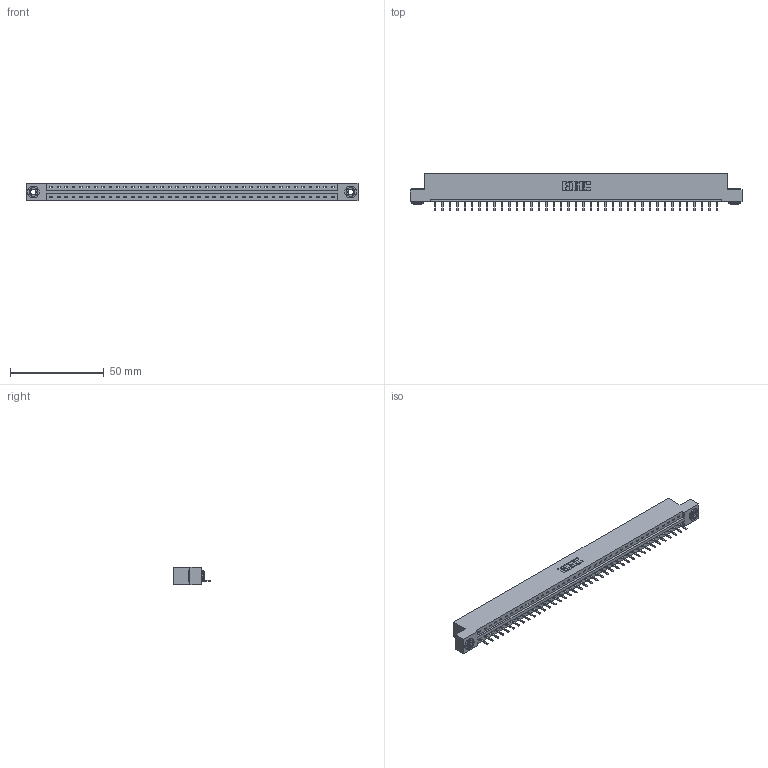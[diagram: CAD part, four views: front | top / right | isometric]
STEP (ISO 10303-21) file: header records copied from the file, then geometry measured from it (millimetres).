
FILE_DESCRIPTION (( 'STEP AP203' ), '1' );
FILE_NAME ('337-039-520-103.STEP', '2019-10-01T18:00:44', ( '' ), ( '' ), 'SwSTEP 2.0', 'SolidWorks 2016', '' );
FILE_SCHEMA (( 'CONFIG_CONTROL_DESIGN' ));
Length unit declared in the file: inch
Products named in the file (4): 345-292-001_345-293-120; 345-250-002_345-250-002-102; 337-039-520-103; 337 Part_Flush Mounting Lugs - 0.156 Dia-TH
Assembly tree (42 placements, depth 2):
  337-039-520-103
    337 Part_Flush Mounting Lugs - 0.156 Dia-TH
    345-292-001_345-293-120  x39
    345-250-002_345-250-002-102  x2
Bounding box: 177.55 x 20.02 x 9.4 mm (x, y, z)
Volume: 18322.6 mm3; surface area: 18745.9 mm2
Topology: 42 solids, 42 shells, 2726 faces, 8031 edges, 5246 vertices
Faces by surface type: plane 1952, cylinder 766, cone 8
Entity records: 30142 total; most frequent: CARTESIAN_POINT 5238, ORIENTED_EDGE 5194, DIRECTION 4437, EDGE_CURVE 2597, LINE 2441, VECTOR 2441, VERTEX_POINT 1726, AXIS2_PLACEMENT_3D 998
